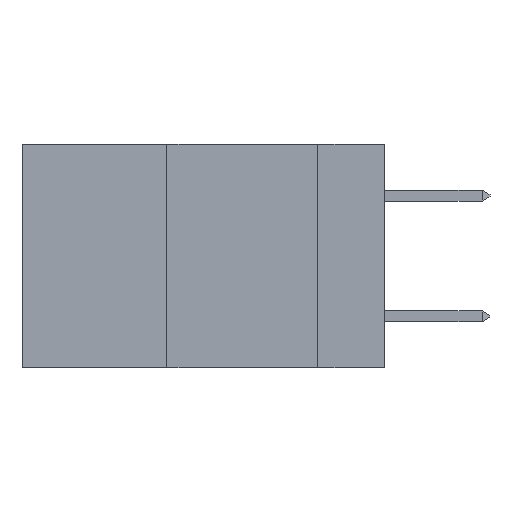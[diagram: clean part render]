
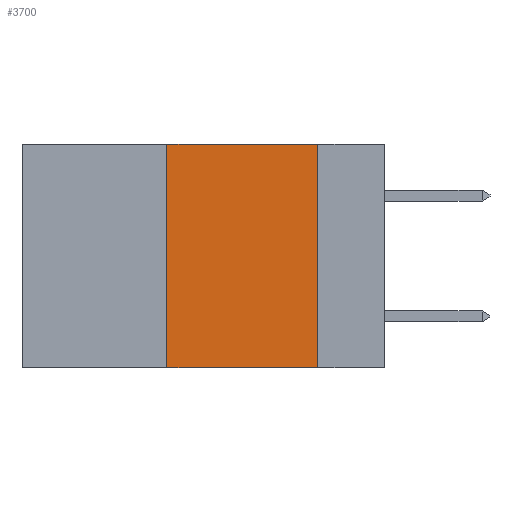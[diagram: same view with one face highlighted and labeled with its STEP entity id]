
A CAD part, left-side view. The second image highlights one B-rep face of the part: STEP entity #3700.
In plain terms, the highlighted planar face has unit normal (-1, 0, 0).
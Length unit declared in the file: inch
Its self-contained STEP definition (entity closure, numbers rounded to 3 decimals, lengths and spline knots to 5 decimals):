
#465 = VERTEX_POINT ( 'NONE', #8625 ) ;
#730 = ORIENTED_EDGE ( 'NONE', *, *, #1233, .F. ) ;
#838 = CARTESIAN_POINT ( 'NONE',  ( 0., 0.6, -0.37 ) ) ;
#1233 = EDGE_CURVE ( 'NONE', #465, #8106, #2863, .T. ) ;
#1643 = VECTOR ( 'NONE', #8494, 39.37008 ) ;
#1695 = CARTESIAN_POINT ( 'NONE',  ( 0., 0.6, 0. ) ) ;
#1842 = DIRECTION ( 'NONE',  ( 0., -1., 0. ) ) ;
#2401 = VECTOR ( 'NONE', #7824, 39.37008 ) ;
#2591 = VECTOR ( 'NONE', #1842, 39.37008 ) ;
#2691 = EDGE_CURVE ( 'NONE', #4769, #8826, #8303, .T. ) ;
#2858 = DIRECTION ( 'NONE',  ( 0., -1., 0. ) ) ;
#2863 = LINE ( 'NONE', #1695, #2591 ) ;
#3062 = ORIENTED_EDGE ( 'NONE', *, *, #3254, .F. ) ;
#3254 = EDGE_CURVE ( 'NONE', #4769, #465, #4690, .T. ) ;
#3700 = ADVANCED_FACE ( 'NONE', ( #5603 ), #10442, .F. ) ;
#3819 = EDGE_CURVE ( 'NONE', #8106, #8826, #6279, .T. ) ;
#4690 = LINE ( 'NONE', #7672, #2401 ) ;
#4769 = VERTEX_POINT ( 'NONE', #9194 ) ;
#5440 = AXIS2_PLACEMENT_3D ( 'NONE', #10530, #10430, #10406 ) ;
#5603 = FACE_OUTER_BOUND ( 'NONE', #9505, .T. ) ;
#5818 = CARTESIAN_POINT ( 'NONE',  ( 0., 0.11, -0.37 ) ) ;
#6279 = LINE ( 'NONE', #8744, #1643 ) ;
#7632 = ORIENTED_EDGE ( 'NONE', *, *, #2691, .T. ) ;
#7672 = CARTESIAN_POINT ( 'NONE',  ( 0., 0.36, 0. ) ) ;
#7824 = DIRECTION ( 'NONE',  ( 0., 0., 1. ) ) ;
#8106 = VERTEX_POINT ( 'NONE', #8972 ) ;
#8303 = LINE ( 'NONE', #838, #10195 ) ;
#8494 = DIRECTION ( 'NONE',  ( 0., 0., -1. ) ) ;
#8625 = CARTESIAN_POINT ( 'NONE',  ( 0., 0.36, 0. ) ) ;
#8744 = CARTESIAN_POINT ( 'NONE',  ( 0., 0.11, 0. ) ) ;
#8826 = VERTEX_POINT ( 'NONE', #5818 ) ;
#8972 = CARTESIAN_POINT ( 'NONE',  ( 0., 0.11, 0. ) ) ;
#9194 = CARTESIAN_POINT ( 'NONE',  ( 0., 0.36, -0.37 ) ) ;
#9505 = EDGE_LOOP ( 'NONE', ( #10534, #730, #3062, #7632 ) ) ;
#10195 = VECTOR ( 'NONE', #2858, 39.37008 ) ;
#10406 = DIRECTION ( 'NONE',  ( 0., 0., -1. ) ) ;
#10430 = DIRECTION ( 'NONE',  ( 1., 0., 0. ) ) ;
#10442 = PLANE ( 'NONE',  #5440 ) ;
#10530 = CARTESIAN_POINT ( 'NONE',  ( 0., 0.6, 0. ) ) ;
#10534 = ORIENTED_EDGE ( 'NONE', *, *, #3819, .F. ) ;
